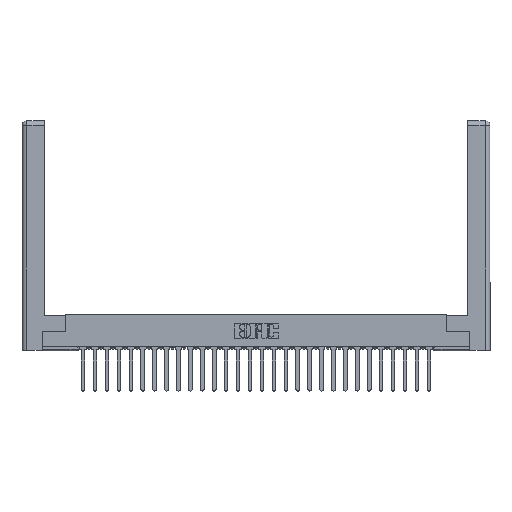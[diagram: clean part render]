
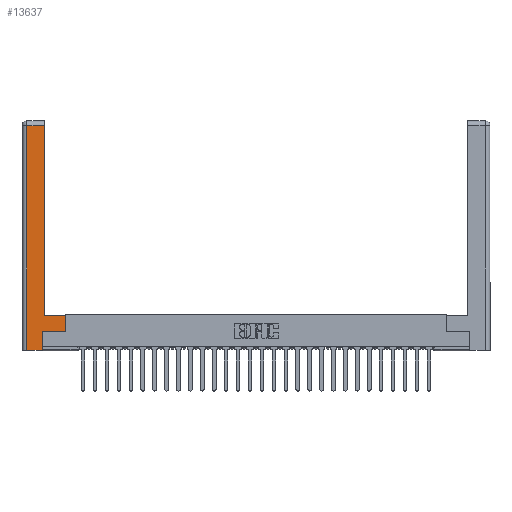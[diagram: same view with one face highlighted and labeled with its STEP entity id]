
A CAD part, top view. The second image highlights one B-rep face of the part: STEP entity #13637.
In plain terms, the highlighted planar face has unit normal (0, 0, 1).
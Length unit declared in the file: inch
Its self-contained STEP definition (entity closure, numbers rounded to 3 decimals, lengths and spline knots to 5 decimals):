
#479 = LINE ( 'NONE', #9961, #4438 ) ;
#1132 = CARTESIAN_POINT ( 'NONE',  ( 0.265, 0.245, 0. ) ) ;
#1188 = FACE_OUTER_BOUND ( 'NONE', #2688, .T. ) ;
#2688 = EDGE_LOOP ( 'NONE', ( #13574, #27557, #20562, #28947, #25053, #3109, #21106, #11085 ) ) ;
#3109 = ORIENTED_EDGE ( 'NONE', *, *, #27430, .T. ) ;
#4198 = VECTOR ( 'NONE', #22051, 39.37008 ) ;
#4353 = VERTEX_POINT ( 'NONE', #29013 ) ;
#4365 = LINE ( 'NONE', #28327, #9886 ) ;
#4438 = VECTOR ( 'NONE', #6228, 39.37008 ) ;
#4978 = EDGE_CURVE ( 'NONE', #28659, #27803, #20746, .T. ) ;
#5431 = VERTEX_POINT ( 'NONE', #8055 ) ;
#5861 = CARTESIAN_POINT ( 'NONE',  ( 0., 0., 0. ) ) ;
#6228 = DIRECTION ( 'NONE',  ( 0., 1., 0. ) ) ;
#6523 = EDGE_CURVE ( 'NONE', #25954, #28659, #26288, .T. ) ;
#6755 = EDGE_CURVE ( 'NONE', #7695, #5431, #22394, .T. ) ;
#7104 = VERTEX_POINT ( 'NONE', #29068 ) ;
#7631 = VECTOR ( 'NONE', #24880, 39.37008 ) ;
#7695 = VERTEX_POINT ( 'NONE', #22726 ) ;
#8055 = CARTESIAN_POINT ( 'NONE',  ( 0.295, 0.45, 0. ) ) ;
#8905 = EDGE_CURVE ( 'NONE', #4353, #7695, #479, .T. ) ;
#9389 = CARTESIAN_POINT ( 'NONE',  ( 0.0615, 2.94, 0. ) ) ;
#9492 = CARTESIAN_POINT ( 'NONE',  ( 0.0615, 0., 0. ) ) ;
#9886 = VECTOR ( 'NONE', #23219, 39.37008 ) ;
#9961 = CARTESIAN_POINT ( 'NONE',  ( 0.565, 0.45, 0. ) ) ;
#10608 = VECTOR ( 'NONE', #30241, 39.37008 ) ;
#10748 = CARTESIAN_POINT ( 'NONE',  ( 0.265, 0., 0. ) ) ;
#11085 = ORIENTED_EDGE ( 'NONE', *, *, #6755, .T. ) ;
#12181 = CARTESIAN_POINT ( 'NONE',  ( 0.565, 0.245, 0. ) ) ;
#12548 = CARTESIAN_POINT ( 'NONE',  ( 0.0615, 2.94, 0. ) ) ;
#12882 = CARTESIAN_POINT ( 'NONE',  ( 0.265, 0.245, 0. ) ) ;
#13574 = ORIENTED_EDGE ( 'NONE', *, *, #22521, .T. ) ;
#13637 = ADVANCED_FACE ( 'NONE', ( #1188 ), #29878, .F. ) ;
#13973 = DIRECTION ( 'NONE',  ( -1., 0., 0. ) ) ;
#14483 = DIRECTION ( 'NONE',  ( 0., -1., 0. ) ) ;
#14751 = VECTOR ( 'NONE', #14483, 39.37008 ) ;
#15374 = DIRECTION ( 'NONE',  ( 0., 0., -1. ) ) ;
#18907 = CARTESIAN_POINT ( 'NONE',  ( 0.265, 0., 0. ) ) ;
#20562 = ORIENTED_EDGE ( 'NONE', *, *, #6523, .T. ) ;
#20746 = LINE ( 'NONE', #10748, #10608 ) ;
#20887 = VECTOR ( 'NONE', #25183, 39.37008 ) ;
#21106 = ORIENTED_EDGE ( 'NONE', *, *, #8905, .T. ) ;
#22051 = DIRECTION ( 'NONE',  ( -1., 0., 0. ) ) ;
#22394 = LINE ( 'NONE', #27214, #7631 ) ;
#22487 = VECTOR ( 'NONE', #26502, 39.37008 ) ;
#22521 = EDGE_CURVE ( 'NONE', #5431, #7104, #4365, .T. ) ;
#22553 = LINE ( 'NONE', #12882, #20887 ) ;
#22726 = CARTESIAN_POINT ( 'NONE',  ( 0.565, 0.45, 0. ) ) ;
#22746 = EDGE_CURVE ( 'NONE', #27803, #24446, #22553, .T. ) ;
#23219 = DIRECTION ( 'NONE',  ( 0., 1., 0. ) ) ;
#23878 = LINE ( 'NONE', #12181, #22487 ) ;
#24388 = LINE ( 'NONE', #12548, #4198 ) ;
#24446 = VERTEX_POINT ( 'NONE', #1132 ) ;
#24880 = DIRECTION ( 'NONE',  ( -1., 0., 0. ) ) ;
#25053 = ORIENTED_EDGE ( 'NONE', *, *, #22746, .T. ) ;
#25183 = DIRECTION ( 'NONE',  ( 0., 1., 0. ) ) ;
#25954 = VERTEX_POINT ( 'NONE', #9389 ) ;
#26000 = CARTESIAN_POINT ( 'NONE',  ( 0.0615, 0., 0. ) ) ;
#26288 = LINE ( 'NONE', #26000, #14751 ) ;
#26502 = DIRECTION ( 'NONE',  ( 1., 0., 0. ) ) ;
#27214 = CARTESIAN_POINT ( 'NONE',  ( 0.295, 0.45, 0. ) ) ;
#27430 = EDGE_CURVE ( 'NONE', #24446, #4353, #23878, .T. ) ;
#27450 = AXIS2_PLACEMENT_3D ( 'NONE', #5861, #15374, #13973 ) ;
#27557 = ORIENTED_EDGE ( 'NONE', *, *, #29272, .T. ) ;
#27803 = VERTEX_POINT ( 'NONE', #18907 ) ;
#28327 = CARTESIAN_POINT ( 'NONE',  ( 0.295, 3., 0. ) ) ;
#28659 = VERTEX_POINT ( 'NONE', #9492 ) ;
#28947 = ORIENTED_EDGE ( 'NONE', *, *, #4978, .T. ) ;
#29013 = CARTESIAN_POINT ( 'NONE',  ( 0.565, 0.245, 0. ) ) ;
#29068 = CARTESIAN_POINT ( 'NONE',  ( 0.295, 2.94, 0. ) ) ;
#29272 = EDGE_CURVE ( 'NONE', #7104, #25954, #24388, .T. ) ;
#29878 = PLANE ( 'NONE',  #27450 ) ;
#30241 = DIRECTION ( 'NONE',  ( 1., 0., 0. ) ) ;
